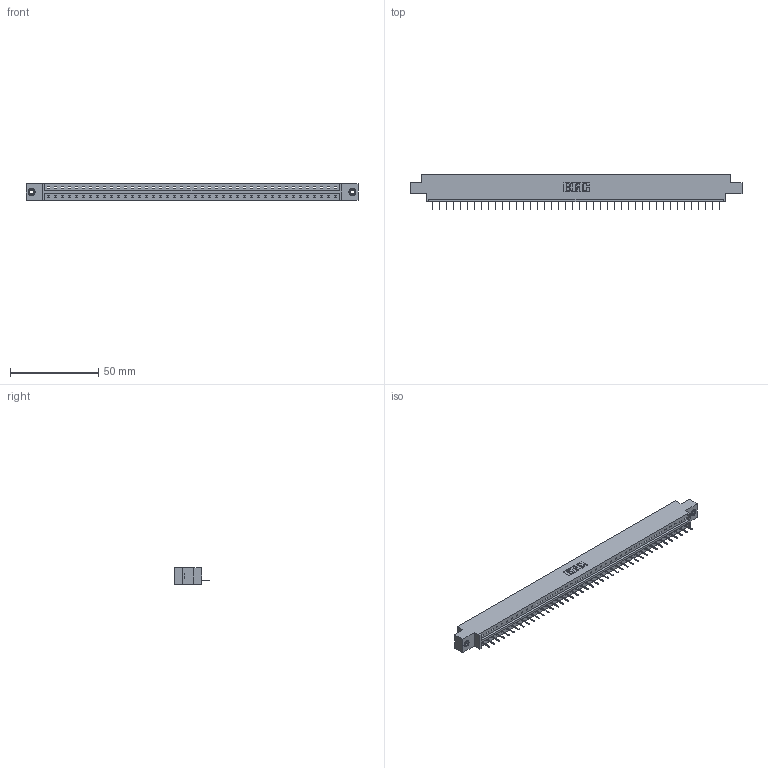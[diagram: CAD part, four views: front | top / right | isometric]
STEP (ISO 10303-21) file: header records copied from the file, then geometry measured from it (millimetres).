
FILE_DESCRIPTION (( 'STEP AP203' ), '1' );
FILE_NAME ('333-042-524-608.STEP', '2018-08-03T18:45:34', ( '' ), ( '' ), 'SwSTEP 2.0', 'SolidWorks 2016', '' );
FILE_SCHEMA (( 'CONFIG_CONTROL_DESIGN' ));
Length unit declared in the file: inch
Products named in the file (4): 333 Part_Offset - .156 Dia - TI; 345-292-001_345-293-124; 345-250-001_345-250-003-102; 333-042-524-608
Assembly tree (45 placements, depth 2):
  333-042-524-608
    333 Part_Offset - .156 Dia - TI
    345-292-001_345-293-124  x42
    345-250-001_345-250-003-102  x2
Bounding box: 187.96 x 19.69 x 9.4 mm (x, y, z)
Volume: 18513.9 mm3; surface area: 19685.4 mm2
Topology: 45 solids, 45 shells, 2782 faces, 8019 edges, 5170 vertices
Faces by surface type: plane 2122, cylinder 644, cone 12, torus 4
Entity records: 27068 total; most frequent: CARTESIAN_POINT 4651, ORIENTED_EDGE 4622, DIRECTION 3957, EDGE_CURVE 2311, VECTOR 2167, LINE 2167, VERTEX_POINT 1532, AXIS2_PLACEMENT_3D 895
